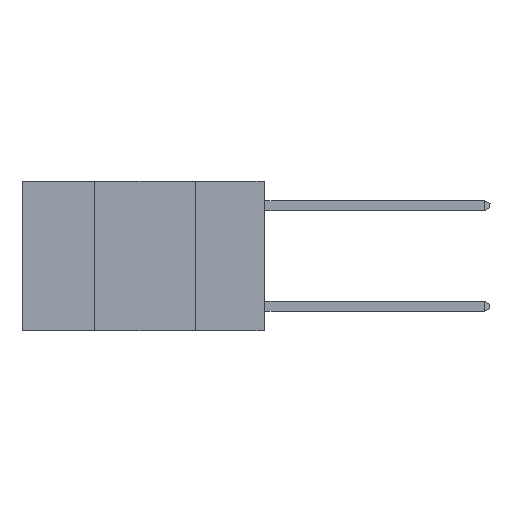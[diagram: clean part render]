
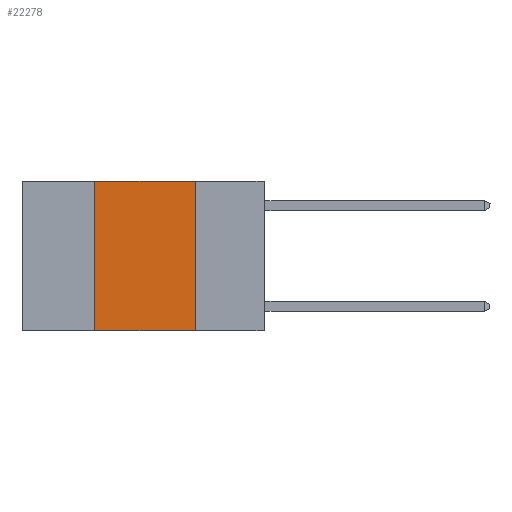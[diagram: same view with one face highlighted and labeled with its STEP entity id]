
A CAD part, left-side view. The second image highlights one B-rep face of the part: STEP entity #22278.
In plain terms, the highlighted planar face has unit normal (-1, 0, 0).
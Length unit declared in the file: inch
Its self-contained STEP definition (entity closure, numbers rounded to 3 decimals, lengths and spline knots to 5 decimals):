
#873 = CARTESIAN_POINT ( 'NONE',  ( 0., 0.42, 0. ) ) ;
#1217 = CARTESIAN_POINT ( 'NONE',  ( 0., 0.6, 0. ) ) ;
#1505 = CARTESIAN_POINT ( 'NONE',  ( 0., 0.6, 0. ) ) ;
#3111 = VECTOR ( 'NONE', #9023, 39.37008 ) ;
#4039 = EDGE_CURVE ( 'NONE', #14868, #19645, #19036, .T. ) ;
#4855 = EDGE_CURVE ( 'NONE', #23009, #12078, #16617, .T. ) ;
#7145 = VECTOR ( 'NONE', #9212, 39.37008 ) ;
#8912 = VECTOR ( 'NONE', #13656, 39.37008 ) ;
#9023 = DIRECTION ( 'NONE',  ( 0., 0., 1. ) ) ;
#9212 = DIRECTION ( 'NONE',  ( 0., -1., 0. ) ) ;
#9488 = DIRECTION ( 'NONE',  ( 0., 0., -1. ) ) ;
#9737 = DIRECTION ( 'NONE',  ( 1., 0., 0. ) ) ;
#10317 = ORIENTED_EDGE ( 'NONE', *, *, #4039, .F. ) ;
#10465 = DIRECTION ( 'NONE',  ( 0., -1., 0. ) ) ;
#11372 = CARTESIAN_POINT ( 'NONE',  ( 0., 0.17, 0. ) ) ;
#11460 = CARTESIAN_POINT ( 'NONE',  ( 0., 0.17, 0. ) ) ;
#12078 = VERTEX_POINT ( 'NONE', #23545 ) ;
#13656 = DIRECTION ( 'NONE',  ( 0., 0., -1. ) ) ;
#14229 = EDGE_CURVE ( 'NONE', #23009, #14868, #18971, .T. ) ;
#14274 = AXIS2_PLACEMENT_3D ( 'NONE', #1505, #9737, #9488 ) ;
#14868 = VERTEX_POINT ( 'NONE', #21791 ) ;
#15798 = FACE_OUTER_BOUND ( 'NONE', #23301, .T. ) ;
#16153 = ORIENTED_EDGE ( 'NONE', *, *, #24761, .F. ) ;
#16617 = LINE ( 'NONE', #24160, #19819 ) ;
#18971 = LINE ( 'NONE', #873, #3111 ) ;
#19036 = LINE ( 'NONE', #1217, #7145 ) ;
#19243 = ORIENTED_EDGE ( 'NONE', *, *, #14229, .F. ) ;
#19311 = PLANE ( 'NONE',  #14274 ) ;
#19645 = VERTEX_POINT ( 'NONE', #11372 ) ;
#19819 = VECTOR ( 'NONE', #10465, 39.37008 ) ;
#21791 = CARTESIAN_POINT ( 'NONE',  ( 0., 0.42, 0. ) ) ;
#22089 = ORIENTED_EDGE ( 'NONE', *, *, #4855, .T. ) ;
#22278 = ADVANCED_FACE ( 'NONE', ( #15798 ), #19311, .F. ) ;
#22882 = CARTESIAN_POINT ( 'NONE',  ( 0., 0.42, -0.37 ) ) ;
#23009 = VERTEX_POINT ( 'NONE', #22882 ) ;
#23301 = EDGE_LOOP ( 'NONE', ( #16153, #10317, #19243, #22089 ) ) ;
#23545 = CARTESIAN_POINT ( 'NONE',  ( 0., 0.17, -0.37 ) ) ;
#24160 = CARTESIAN_POINT ( 'NONE',  ( 0., 0.6, -0.37 ) ) ;
#24761 = EDGE_CURVE ( 'NONE', #19645, #12078, #25187, .T. ) ;
#25187 = LINE ( 'NONE', #11460, #8912 ) ;
